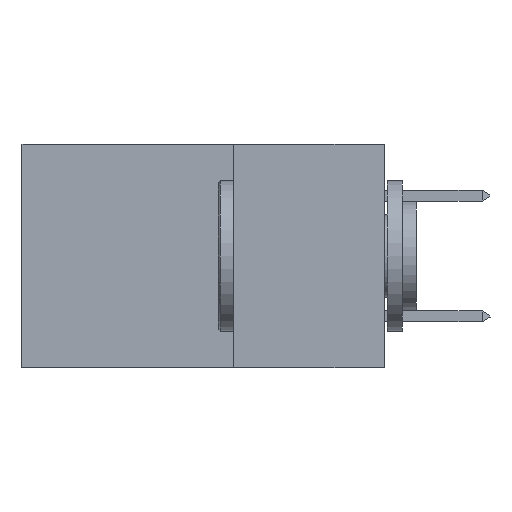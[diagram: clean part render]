
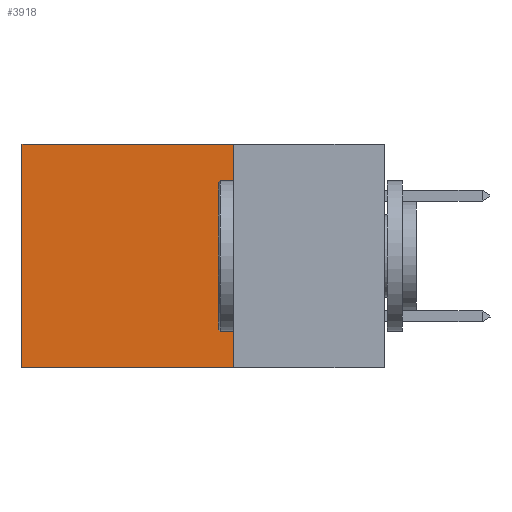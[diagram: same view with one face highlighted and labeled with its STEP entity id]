
A CAD part, left-side view. The second image highlights one B-rep face of the part: STEP entity #3918.
In plain terms, the highlighted planar face has unit normal (-1, 0, 0).
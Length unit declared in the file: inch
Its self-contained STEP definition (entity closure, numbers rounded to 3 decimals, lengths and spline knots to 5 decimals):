
#45 = CARTESIAN_POINT ( 'NONE',  ( 0.2875, 0.25, 0. ) ) ;
#351 = EDGE_LOOP ( 'NONE', ( #1604, #5166, #21603, #10713 ) ) ;
#857 = CARTESIAN_POINT ( 'NONE',  ( 0.2875, 0.6, 0. ) ) ;
#1604 = ORIENTED_EDGE ( 'NONE', *, *, #13899, .T. ) ;
#3564 = VERTEX_POINT ( 'NONE', #10646 ) ;
#3918 = ADVANCED_FACE ( 'NONE', ( #21440 ), #7974, .F. ) ;
#4249 = DIRECTION ( 'NONE',  ( 0., 0., -1. ) ) ;
#4494 = VERTEX_POINT ( 'NONE', #45 ) ;
#5166 = ORIENTED_EDGE ( 'NONE', *, *, #23097, .F. ) ;
#5789 = CARTESIAN_POINT ( 'NONE',  ( 0.2875, 0.25, -0.37 ) ) ;
#7620 = EDGE_CURVE ( 'NONE', #4494, #11354, #9402, .T. ) ;
#7974 = PLANE ( 'NONE',  #16701 ) ;
#8011 = VECTOR ( 'NONE', #22515, 39.37008 ) ;
#9402 = LINE ( 'NONE', #11519, #18181 ) ;
#9765 = DIRECTION ( 'NONE',  ( 0., 0., -1. ) ) ;
#10646 = CARTESIAN_POINT ( 'NONE',  ( 0.2875, 0.25, -0.37 ) ) ;
#10713 = ORIENTED_EDGE ( 'NONE', *, *, #7620, .T. ) ;
#11354 = VERTEX_POINT ( 'NONE', #20162 ) ;
#11519 = CARTESIAN_POINT ( 'NONE',  ( 0.2875, 0.25, 0. ) ) ;
#11590 = LINE ( 'NONE', #20472, #18098 ) ;
#12847 = VECTOR ( 'NONE', #14805, 39.37008 ) ;
#13899 = EDGE_CURVE ( 'NONE', #11354, #19530, #18175, .T. ) ;
#14805 = DIRECTION ( 'NONE',  ( 0., 1., 0. ) ) ;
#15374 = LINE ( 'NONE', #5789, #12847 ) ;
#16701 = AXIS2_PLACEMENT_3D ( 'NONE', #22141, #20500, #9765 ) ;
#18098 = VECTOR ( 'NONE', #4249, 39.37008 ) ;
#18175 = LINE ( 'NONE', #857, #8011 ) ;
#18181 = VECTOR ( 'NONE', #19006, 39.37008 ) ;
#18909 = EDGE_CURVE ( 'NONE', #4494, #3564, #11590, .T. ) ;
#19006 = DIRECTION ( 'NONE',  ( 0., 1., 0. ) ) ;
#19530 = VERTEX_POINT ( 'NONE', #22323 ) ;
#20162 = CARTESIAN_POINT ( 'NONE',  ( 0.2875, 0.6, 0. ) ) ;
#20472 = CARTESIAN_POINT ( 'NONE',  ( 0.2875, 0.25, 0. ) ) ;
#20500 = DIRECTION ( 'NONE',  ( 1., 0., 0. ) ) ;
#21440 = FACE_OUTER_BOUND ( 'NONE', #351, .T. ) ;
#21603 = ORIENTED_EDGE ( 'NONE', *, *, #18909, .F. ) ;
#22141 = CARTESIAN_POINT ( 'NONE',  ( 0.2875, 0.25, 0. ) ) ;
#22323 = CARTESIAN_POINT ( 'NONE',  ( 0.2875, 0.6, -0.37 ) ) ;
#22515 = DIRECTION ( 'NONE',  ( 0., 0., -1. ) ) ;
#23097 = EDGE_CURVE ( 'NONE', #3564, #19530, #15374, .T. ) ;
